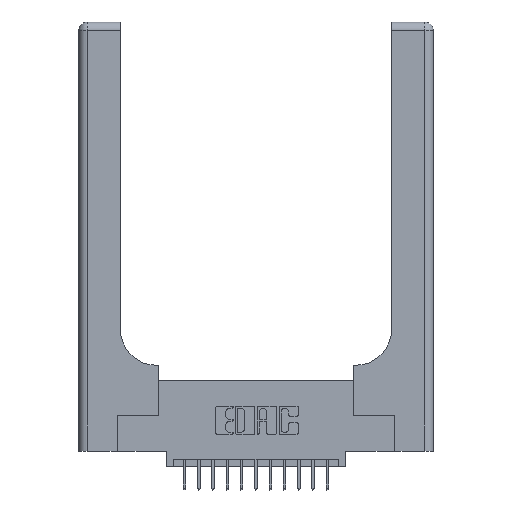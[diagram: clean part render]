
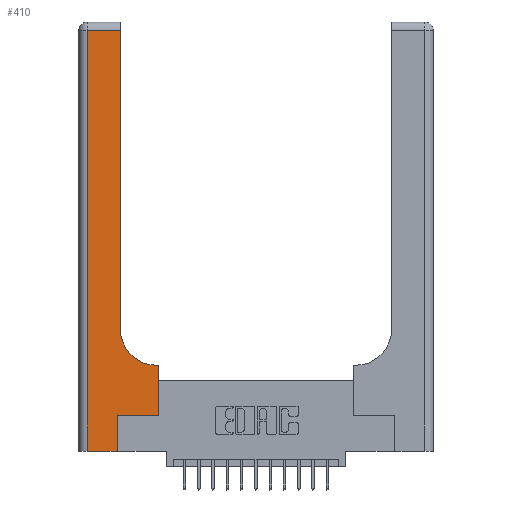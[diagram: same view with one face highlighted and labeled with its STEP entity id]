
A CAD part, top view. The second image highlights one B-rep face of the part: STEP entity #410.
In plain terms, the highlighted planar face has unit normal (0, 0, 1).
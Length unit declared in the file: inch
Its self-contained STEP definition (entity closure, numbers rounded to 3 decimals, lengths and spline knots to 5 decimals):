
#399 = CARTESIAN_POINT ( 'NONE',  ( 0., 0., 0.37 ) ) ;
#410 = ADVANCED_FACE ( 'NONE', ( #10232 ), #9791, .F. ) ;
#473 = CARTESIAN_POINT ( 'NONE',  ( 0.269, 0., 0.37 ) ) ;
#1262 = CARTESIAN_POINT ( 'NONE',  ( 0.2915, 2.94, 0.37 ) ) ;
#1266 = DIRECTION ( 'NONE',  ( 0., 0., -1. ) ) ;
#1404 = VECTOR ( 'NONE', #10406, 39.37008 ) ;
#2068 = VERTEX_POINT ( 'NONE', #13831 ) ;
#2181 = LINE ( 'NONE', #6697, #11611 ) ;
#2210 = EDGE_CURVE ( 'NONE', #11276, #6047, #15048, .T. ) ;
#2585 = EDGE_CURVE ( 'NONE', #2068, #12296, #5329, .T. ) ;
#2736 = DIRECTION ( 'NONE',  ( -1., 0., 0. ) ) ;
#3169 = CARTESIAN_POINT ( 'NONE',  ( 0.5585, 0.25, 0.37 ) ) ;
#3855 = ORIENTED_EDGE ( 'NONE', *, *, #2210, .T. ) ;
#4020 = CARTESIAN_POINT ( 'NONE',  ( 0., 2.94, 0.37 ) ) ;
#4023 = EDGE_CURVE ( 'NONE', #6047, #16047, #16953, .T. ) ;
#4252 = DIRECTION ( 'NONE',  ( 0., 0., -1. ) ) ;
#4339 = LINE ( 'NONE', #3169, #16461 ) ;
#4754 = VECTOR ( 'NONE', #7941, 39.37008 ) ;
#5287 = DIRECTION ( 'NONE',  ( -1., 0., 0. ) ) ;
#5329 = LINE ( 'NONE', #13251, #10576 ) ;
#5441 = ORIENTED_EDGE ( 'NONE', *, *, #17945, .T. ) ;
#6047 = VERTEX_POINT ( 'NONE', #8690 ) ;
#6254 = CARTESIAN_POINT ( 'NONE',  ( 0.06, 0., 0.37 ) ) ;
#6320 = CARTESIAN_POINT ( 'NONE',  ( 0.5585, 0.6, 0.37 ) ) ;
#6697 = CARTESIAN_POINT ( 'NONE',  ( 0.2915, 0.6, 0.37 ) ) ;
#6887 = ORIENTED_EDGE ( 'NONE', *, *, #4023, .T. ) ;
#7076 = LINE ( 'NONE', #4020, #9284 ) ;
#7170 = LINE ( 'NONE', #12126, #4754 ) ;
#7459 = EDGE_CURVE ( 'NONE', #12296, #15709, #13355, .T. ) ;
#7532 = ORIENTED_EDGE ( 'NONE', *, *, #2585, .T. ) ;
#7584 = ORIENTED_EDGE ( 'NONE', *, *, #8986, .T. ) ;
#7690 = DIRECTION ( 'NONE',  ( 1., 0., 0. ) ) ;
#7941 = DIRECTION ( 'NONE',  ( 1., 0., 0. ) ) ;
#8063 = EDGE_CURVE ( 'NONE', #12294, #8490, #4339, .T. ) ;
#8266 = DIRECTION ( 'NONE',  ( 0., 1., 0. ) ) ;
#8384 = CARTESIAN_POINT ( 'NONE',  ( 0., 3., 0.37 ) ) ;
#8490 = VERTEX_POINT ( 'NONE', #6320 ) ;
#8690 = CARTESIAN_POINT ( 'NONE',  ( 0.2915, 0.85, 0.37 ) ) ;
#8986 = EDGE_CURVE ( 'NONE', #15017, #12294, #7170, .T. ) ;
#9284 = VECTOR ( 'NONE', #10886, 39.37008 ) ;
#9358 = CARTESIAN_POINT ( 'NONE',  ( 0.5415, 0.85, 0.37 ) ) ;
#9791 = PLANE ( 'NONE',  #12011 ) ;
#9955 = EDGE_CURVE ( 'NONE', #15709, #15017, #16819, .T. ) ;
#10000 = CARTESIAN_POINT ( 'NONE',  ( 0.269, 0.25, 0.37 ) ) ;
#10133 = ORIENTED_EDGE ( 'NONE', *, *, #11027, .T. ) ;
#10232 = FACE_OUTER_BOUND ( 'NONE', #15148, .T. ) ;
#10406 = DIRECTION ( 'NONE',  ( 0., 1., 0. ) ) ;
#10576 = VECTOR ( 'NONE', #16675, 39.37008 ) ;
#10886 = DIRECTION ( 'NONE',  ( -1., 0., 0. ) ) ;
#11027 = EDGE_CURVE ( 'NONE', #16047, #2068, #7076, .T. ) ;
#11276 = VERTEX_POINT ( 'NONE', #16080 ) ;
#11611 = VECTOR ( 'NONE', #5287, 39.37008 ) ;
#12011 = AXIS2_PLACEMENT_3D ( 'NONE', #8384, #1266, #2736 ) ;
#12126 = CARTESIAN_POINT ( 'NONE',  ( 0.269, 0.25, 0.37 ) ) ;
#12294 = VERTEX_POINT ( 'NONE', #16065 ) ;
#12296 = VERTEX_POINT ( 'NONE', #6254 ) ;
#13201 = VECTOR ( 'NONE', #8266, 39.37008 ) ;
#13230 = DIRECTION ( 'NONE',  ( 1., 0., 0. ) ) ;
#13251 = CARTESIAN_POINT ( 'NONE',  ( 0.06, 3., 0.37 ) ) ;
#13355 = LINE ( 'NONE', #399, #14473 ) ;
#13831 = CARTESIAN_POINT ( 'NONE',  ( 0.06, 2.94, 0.37 ) ) ;
#13911 = CARTESIAN_POINT ( 'NONE',  ( 0.2915, 3., 0.37 ) ) ;
#14375 = AXIS2_PLACEMENT_3D ( 'NONE', #9358, #4252, #7690 ) ;
#14433 = CARTESIAN_POINT ( 'NONE',  ( 0.269, 0., 0.37 ) ) ;
#14473 = VECTOR ( 'NONE', #13230, 39.37008 ) ;
#14697 = ORIENTED_EDGE ( 'NONE', *, *, #8063, .T. ) ;
#15017 = VERTEX_POINT ( 'NONE', #10000 ) ;
#15048 = CIRCLE ( 'NONE', #14375, 0.25 ) ;
#15148 = EDGE_LOOP ( 'NONE', ( #6887, #10133, #7532, #16624, #15587, #7584, #14697, #5441, #3855 ) ) ;
#15587 = ORIENTED_EDGE ( 'NONE', *, *, #9955, .T. ) ;
#15709 = VERTEX_POINT ( 'NONE', #473 ) ;
#16047 = VERTEX_POINT ( 'NONE', #1262 ) ;
#16065 = CARTESIAN_POINT ( 'NONE',  ( 0.5585, 0.25, 0.37 ) ) ;
#16080 = CARTESIAN_POINT ( 'NONE',  ( 0.5415, 0.6, 0.37 ) ) ;
#16461 = VECTOR ( 'NONE', #18032, 39.37008 ) ;
#16624 = ORIENTED_EDGE ( 'NONE', *, *, #7459, .T. ) ;
#16675 = DIRECTION ( 'NONE',  ( 0., -1., 0. ) ) ;
#16819 = LINE ( 'NONE', #14433, #1404 ) ;
#16953 = LINE ( 'NONE', #13911, #13201 ) ;
#17945 = EDGE_CURVE ( 'NONE', #8490, #11276, #2181, .T. ) ;
#18032 = DIRECTION ( 'NONE',  ( 0., 1., 0. ) ) ;
